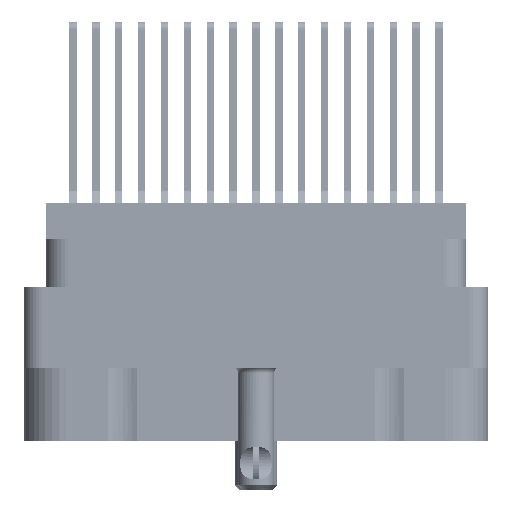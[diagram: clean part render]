
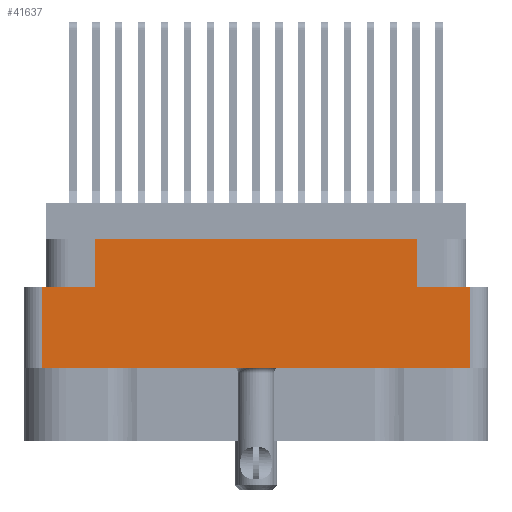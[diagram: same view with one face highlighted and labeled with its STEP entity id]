
A CAD part, left-side view. The second image highlights one B-rep face of the part: STEP entity #41637.
In plain terms, the highlighted planar face has unit normal (-1, 0, 0).
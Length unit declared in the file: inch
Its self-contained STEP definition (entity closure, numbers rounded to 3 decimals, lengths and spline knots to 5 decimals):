
#308 = CARTESIAN_POINT ( 'NONE',  ( -1.375, -0.7005, -0.274 ) ) ;
#490 = LINE ( 'NONE', #55395, #68417 ) ;
#556 = CARTESIAN_POINT ( 'NONE',  ( -1.375, 0., -0.274 ) ) ;
#1209 = CARTESIAN_POINT ( 'NONE',  ( -1.375, -0.5285, -0.117 ) ) ;
#1449 = ORIENTED_EDGE ( 'NONE', *, *, #76946, .F. ) ;
#1513 = VERTEX_POINT ( 'NONE', #21404 ) ;
#2984 = CARTESIAN_POINT ( 'NONE',  ( -1.375, 0.7005, -0.274 ) ) ;
#3354 = VERTEX_POINT ( 'NONE', #34734 ) ;
#3798 = VECTOR ( 'NONE', #98557, 39.37008 ) ;
#7378 = ORIENTED_EDGE ( 'NONE', *, *, #33023, .F. ) ;
#7645 = DIRECTION ( 'NONE',  ( 0., 0., -1. ) ) ;
#9519 = CARTESIAN_POINT ( 'NONE',  ( -1.375, -0.5285, -0.274 ) ) ;
#10165 = CARTESIAN_POINT ( 'NONE',  ( -1.375, 0.5285, -0.274 ) ) ;
#12204 = VECTOR ( 'NONE', #26014, 39.37008 ) ;
#12673 = ORIENTED_EDGE ( 'NONE', *, *, #25770, .T. ) ;
#13527 = VECTOR ( 'NONE', #54420, 39.37008 ) ;
#14578 = ORIENTED_EDGE ( 'NONE', *, *, #49800, .T. ) ;
#15795 = LINE ( 'NONE', #556, #12204 ) ;
#19615 = LINE ( 'NONE', #90463, #3798 ) ;
#20518 = CARTESIAN_POINT ( 'NONE',  ( -1.375, 0., -0.274 ) ) ;
#21404 = CARTESIAN_POINT ( 'NONE',  ( -1.375, 0.5285, -0.117 ) ) ;
#23799 = VECTOR ( 'NONE', #55685, 39.37008 ) ;
#25770 = EDGE_CURVE ( 'NONE', #91467, #66102, #19615, .T. ) ;
#25808 = FACE_OUTER_BOUND ( 'NONE', #97744, .T. ) ;
#26014 = DIRECTION ( 'NONE',  ( 0., -1., 0. ) ) ;
#30093 = ORIENTED_EDGE ( 'NONE', *, *, #85624, .F. ) ;
#31630 = CARTESIAN_POINT ( 'NONE',  ( -1.375, 0.5285, -0.274 ) ) ;
#33023 = EDGE_CURVE ( 'NONE', #93878, #1513, #48090, .T. ) ;
#33851 = CARTESIAN_POINT ( 'NONE',  ( -1.375, 0., -0.54 ) ) ;
#34239 = ORIENTED_EDGE ( 'NONE', *, *, #65347, .T. ) ;
#34734 = CARTESIAN_POINT ( 'NONE',  ( -1.375, -0.7005, -0.54 ) ) ;
#36044 = LINE ( 'NONE', #33851, #54325 ) ;
#36830 = DIRECTION ( 'NONE',  ( 0., -1., 0. ) ) ;
#37040 = EDGE_CURVE ( 'NONE', #58083, #93878, #60705, .T. ) ;
#39190 = VERTEX_POINT ( 'NONE', #308 ) ;
#40018 = VECTOR ( 'NONE', #81683, 39.37008 ) ;
#41637 = ADVANCED_FACE ( 'NONE', ( #25808 ), #98407, .T. ) ;
#43652 = CARTESIAN_POINT ( 'NONE',  ( -1.375, 0.7005, -0.54 ) ) ;
#47511 = VECTOR ( 'NONE', #36830, 39.37008 ) ;
#48090 = LINE ( 'NONE', #31630, #23799 ) ;
#49800 = EDGE_CURVE ( 'NONE', #61145, #3354, #36044, .T. ) ;
#51929 = DIRECTION ( 'NONE',  ( 0., 0., 1. ) ) ;
#52495 = ORIENTED_EDGE ( 'NONE', *, *, #66879, .T. ) ;
#54325 = VECTOR ( 'NONE', #57312, 39.37008 ) ;
#54420 = DIRECTION ( 'NONE',  ( 0., 0., 1. ) ) ;
#55395 = CARTESIAN_POINT ( 'NONE',  ( -1.375, 0.7005, -0.78 ) ) ;
#55685 = DIRECTION ( 'NONE',  ( 0., 0., 1. ) ) ;
#57312 = DIRECTION ( 'NONE',  ( 0., -1., 0. ) ) ;
#57838 = ORIENTED_EDGE ( 'NONE', *, *, #37040, .F. ) ;
#58083 = VERTEX_POINT ( 'NONE', #2984 ) ;
#59414 = CARTESIAN_POINT ( 'NONE',  ( -1.375, -0.7625, -0.78 ) ) ;
#60705 = LINE ( 'NONE', #20518, #40018 ) ;
#60719 = DIRECTION ( 'NONE',  ( -1., 0., 0. ) ) ;
#61145 = VERTEX_POINT ( 'NONE', #43652 ) ;
#65347 = EDGE_CURVE ( 'NONE', #58083, #61145, #490, .T. ) ;
#66102 = VERTEX_POINT ( 'NONE', #1209 ) ;
#66879 = EDGE_CURVE ( 'NONE', #3354, #39190, #75404, .T. ) ;
#68417 = VECTOR ( 'NONE', #7645, 39.37008 ) ;
#69847 = AXIS2_PLACEMENT_3D ( 'NONE', #59414, #60719, #51929 ) ;
#72999 = LINE ( 'NONE', #99980, #47511 ) ;
#75404 = LINE ( 'NONE', #94394, #13527 ) ;
#76946 = EDGE_CURVE ( 'NONE', #1513, #66102, #72999, .T. ) ;
#81683 = DIRECTION ( 'NONE',  ( 0., -1., 0. ) ) ;
#85624 = EDGE_CURVE ( 'NONE', #91467, #39190, #15795, .T. ) ;
#90463 = CARTESIAN_POINT ( 'NONE',  ( -1.375, -0.5285, -0.274 ) ) ;
#91467 = VERTEX_POINT ( 'NONE', #9519 ) ;
#93878 = VERTEX_POINT ( 'NONE', #10165 ) ;
#94394 = CARTESIAN_POINT ( 'NONE',  ( -1.375, -0.7005, -0.78 ) ) ;
#97744 = EDGE_LOOP ( 'NONE', ( #57838, #34239, #14578, #52495, #30093, #12673, #1449, #7378 ) ) ;
#98407 = PLANE ( 'NONE',  #69847 ) ;
#98557 = DIRECTION ( 'NONE',  ( 0., 0., 1. ) ) ;
#99980 = CARTESIAN_POINT ( 'NONE',  ( -1.375, 0.7625, -0.117 ) ) ;
